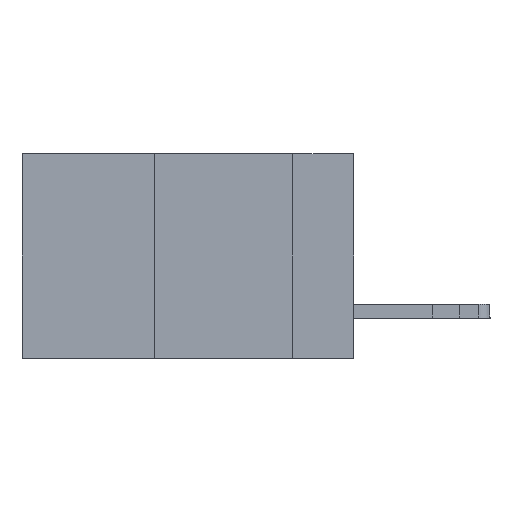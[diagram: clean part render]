
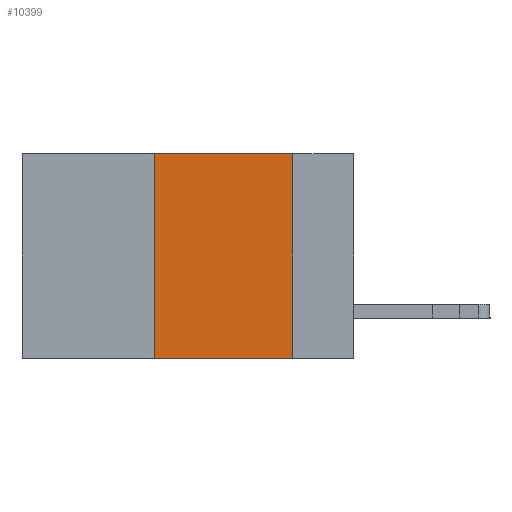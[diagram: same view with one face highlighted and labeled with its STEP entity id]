
A CAD part, left-side view. The second image highlights one B-rep face of the part: STEP entity #10399.
In plain terms, the highlighted planar face has unit normal (-1, 0, 0).
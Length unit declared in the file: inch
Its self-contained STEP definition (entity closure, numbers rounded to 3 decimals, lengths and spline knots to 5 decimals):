
#322 = ORIENTED_EDGE ( 'NONE', *, *, #13880, .F. ) ;
#543 = VERTEX_POINT ( 'NONE', #17577 ) ;
#902 = VECTOR ( 'NONE', #3529, 39.37008 ) ;
#944 = LINE ( 'NONE', #11975, #2684 ) ;
#1253 = DIRECTION ( 'NONE',  ( 0., -1., 0. ) ) ;
#1970 = VERTEX_POINT ( 'NONE', #12563 ) ;
#2606 = AXIS2_PLACEMENT_3D ( 'NONE', #8836, #12838, #15774 ) ;
#2684 = VECTOR ( 'NONE', #16615, 39.37008 ) ;
#3132 = CARTESIAN_POINT ( 'NONE',  ( 0., 0.6, -0.37 ) ) ;
#3529 = DIRECTION ( 'NONE',  ( 0., 0., -1. ) ) ;
#4929 = EDGE_CURVE ( 'NONE', #543, #1970, #14809, .T. ) ;
#6460 = DIRECTION ( 'NONE',  ( 0., 0., 1. ) ) ;
#7839 = EDGE_CURVE ( 'NONE', #1970, #17067, #944, .T. ) ;
#8335 = VECTOR ( 'NONE', #6460, 39.37008 ) ;
#8693 = LINE ( 'NONE', #3132, #9563 ) ;
#8836 = CARTESIAN_POINT ( 'NONE',  ( 0., 0.6, 0. ) ) ;
#9563 = VECTOR ( 'NONE', #1253, 39.37008 ) ;
#10331 = EDGE_LOOP ( 'NONE', ( #322, #16726, #14830, #12858 ) ) ;
#10399 = ADVANCED_FACE ( 'NONE', ( #13654 ), #12901, .F. ) ;
#10862 = EDGE_CURVE ( 'NONE', #543, #15387, #8693, .T. ) ;
#11701 = CARTESIAN_POINT ( 'NONE',  ( 0., 0.11, 0. ) ) ;
#11975 = CARTESIAN_POINT ( 'NONE',  ( 0., 0.6, 0. ) ) ;
#12551 = CARTESIAN_POINT ( 'NONE',  ( 0., 0.11, -0.37 ) ) ;
#12563 = CARTESIAN_POINT ( 'NONE',  ( 0., 0.36, 0. ) ) ;
#12838 = DIRECTION ( 'NONE',  ( 1., 0., 0. ) ) ;
#12858 = ORIENTED_EDGE ( 'NONE', *, *, #10862, .T. ) ;
#12901 = PLANE ( 'NONE',  #2606 ) ;
#13484 = LINE ( 'NONE', #11701, #902 ) ;
#13654 = FACE_OUTER_BOUND ( 'NONE', #10331, .T. ) ;
#13880 = EDGE_CURVE ( 'NONE', #17067, #15387, #13484, .T. ) ;
#14451 = CARTESIAN_POINT ( 'NONE',  ( 0., 0.11, 0. ) ) ;
#14778 = CARTESIAN_POINT ( 'NONE',  ( 0., 0.36, 0. ) ) ;
#14809 = LINE ( 'NONE', #14778, #8335 ) ;
#14830 = ORIENTED_EDGE ( 'NONE', *, *, #4929, .F. ) ;
#15387 = VERTEX_POINT ( 'NONE', #12551 ) ;
#15774 = DIRECTION ( 'NONE',  ( 0., 0., -1. ) ) ;
#16615 = DIRECTION ( 'NONE',  ( 0., -1., 0. ) ) ;
#16726 = ORIENTED_EDGE ( 'NONE', *, *, #7839, .F. ) ;
#17067 = VERTEX_POINT ( 'NONE', #14451 ) ;
#17577 = CARTESIAN_POINT ( 'NONE',  ( 0., 0.36, -0.37 ) ) ;
